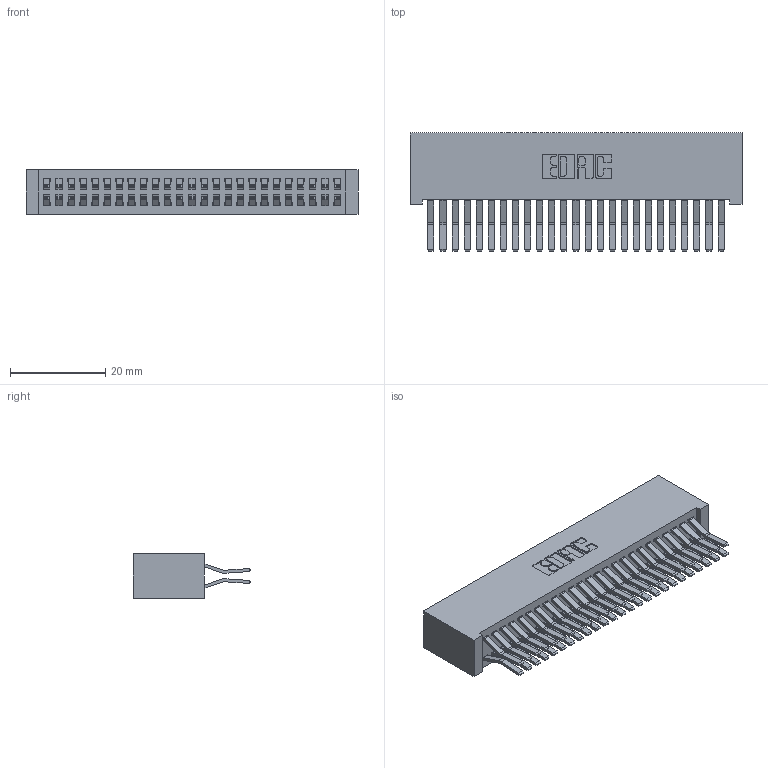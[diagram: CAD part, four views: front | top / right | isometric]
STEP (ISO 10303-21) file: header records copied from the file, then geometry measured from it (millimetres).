
FILE_DESCRIPTION (( 'STEP AP203' ), '1' );
FILE_NAME ('342-050-560-201.STEP', '2019-10-03T00:11:43', ( '' ), ( '' ), 'SwSTEP 2.0', 'SolidWorks 2016', '' );
FILE_SCHEMA (( 'CONFIG_CONTROL_DESIGN' ));
Length unit declared in the file: inch
Products named in the file (3): 342 Part_Lugless; 345-292-001_560 Tail; 342-050-560-201
Assembly tree (51 placements, depth 2):
  342-050-560-201
    342 Part_Lugless
    345-292-001_560 Tail  x50
Bounding box: 69.75 x 24.78 x 9.4 mm (x, y, z)
Volume: 6954.2 mm3; surface area: 12134.2 mm2
Topology: 51 solids, 51 shells, 2802 faces, 8325 edges, 5482 vertices
Faces by surface type: plane 1862, cylinder 940
Entity records: 17961 total; most frequent: CARTESIAN_POINT 2994, ORIENTED_EDGE 2930, DIRECTION 2585, EDGE_CURVE 1465, LINE 1341, VECTOR 1341, VERTEX_POINT 974, AXIS2_PLACEMENT_3D 622
